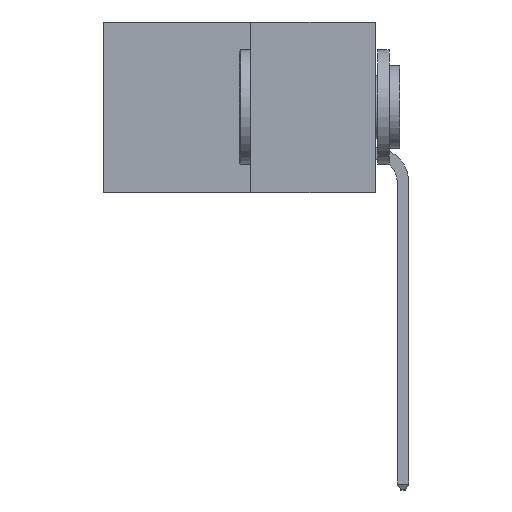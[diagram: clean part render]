
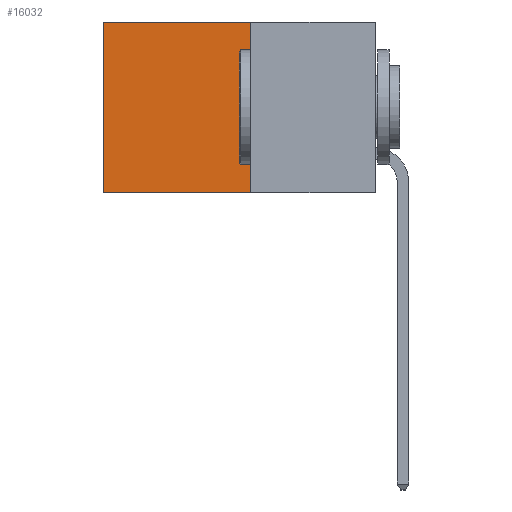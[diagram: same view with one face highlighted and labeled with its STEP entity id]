
A CAD part, left-side view. The second image highlights one B-rep face of the part: STEP entity #16032.
In plain terms, the highlighted planar face has unit normal (-1, 0, 0).
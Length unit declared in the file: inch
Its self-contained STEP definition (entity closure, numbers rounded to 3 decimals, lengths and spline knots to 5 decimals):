
#541 = LINE ( 'NONE', #4605, #21245 ) ;
#1533 = ORIENTED_EDGE ( 'NONE', *, *, #18822, .T. ) ;
#2743 = DIRECTION ( 'NONE',  ( 0., 1., 0. ) ) ;
#3829 = VERTEX_POINT ( 'NONE', #17565 ) ;
#3966 = EDGE_CURVE ( 'NONE', #15182, #3829, #541, .T. ) ;
#4370 = CARTESIAN_POINT ( 'NONE',  ( 0.277, 0.27, 0. ) ) ;
#4605 = CARTESIAN_POINT ( 'NONE',  ( 0.277, 0.27, 0. ) ) ;
#4898 = EDGE_LOOP ( 'NONE', ( #1533, #21500, #24397, #10019 ) ) ;
#4906 = DIRECTION ( 'NONE',  ( 0., 1., 0. ) ) ;
#7687 = CARTESIAN_POINT ( 'NONE',  ( 0.277, 0.27, -0.37 ) ) ;
#8034 = VECTOR ( 'NONE', #11195, 39.37008 ) ;
#8663 = LINE ( 'NONE', #24867, #8034 ) ;
#8833 = FACE_OUTER_BOUND ( 'NONE', #4898, .T. ) ;
#8846 = DIRECTION ( 'NONE',  ( 1., 0., 0. ) ) ;
#8965 = CARTESIAN_POINT ( 'NONE',  ( 0.277, 0.27, -0.37 ) ) ;
#9326 = LINE ( 'NONE', #8965, #13989 ) ;
#10019 = ORIENTED_EDGE ( 'NONE', *, *, #3966, .T. ) ;
#10956 = VERTEX_POINT ( 'NONE', #24191 ) ;
#11195 = DIRECTION ( 'NONE',  ( 0., 0., -1. ) ) ;
#13274 = LINE ( 'NONE', #7687, #23664 ) ;
#13989 = VECTOR ( 'NONE', #4906, 39.37008 ) ;
#14772 = PLANE ( 'NONE',  #25131 ) ;
#15023 = EDGE_CURVE ( 'NONE', #15182, #10956, #13274, .T. ) ;
#15182 = VERTEX_POINT ( 'NONE', #4370 ) ;
#16032 = ADVANCED_FACE ( 'NONE', ( #8833 ), #14772, .F. ) ;
#17565 = CARTESIAN_POINT ( 'NONE',  ( 0.277, 0.59, 0. ) ) ;
#18822 = EDGE_CURVE ( 'NONE', #3829, #19122, #8663, .T. ) ;
#19122 = VERTEX_POINT ( 'NONE', #23858 ) ;
#20669 = CARTESIAN_POINT ( 'NONE',  ( 0.277, 0.27, -0.37 ) ) ;
#21245 = VECTOR ( 'NONE', #2743, 39.37008 ) ;
#21477 = DIRECTION ( 'NONE',  ( 0., 0., -1. ) ) ;
#21500 = ORIENTED_EDGE ( 'NONE', *, *, #24877, .F. ) ;
#22633 = DIRECTION ( 'NONE',  ( 0., 0., -1. ) ) ;
#23664 = VECTOR ( 'NONE', #21477, 39.37008 ) ;
#23858 = CARTESIAN_POINT ( 'NONE',  ( 0.277, 0.59, -0.37 ) ) ;
#24191 = CARTESIAN_POINT ( 'NONE',  ( 0.277, 0.27, -0.37 ) ) ;
#24397 = ORIENTED_EDGE ( 'NONE', *, *, #15023, .F. ) ;
#24867 = CARTESIAN_POINT ( 'NONE',  ( 0.277, 0.59, -0.37 ) ) ;
#24877 = EDGE_CURVE ( 'NONE', #10956, #19122, #9326, .T. ) ;
#25131 = AXIS2_PLACEMENT_3D ( 'NONE', #20669, #8846, #22633 ) ;
